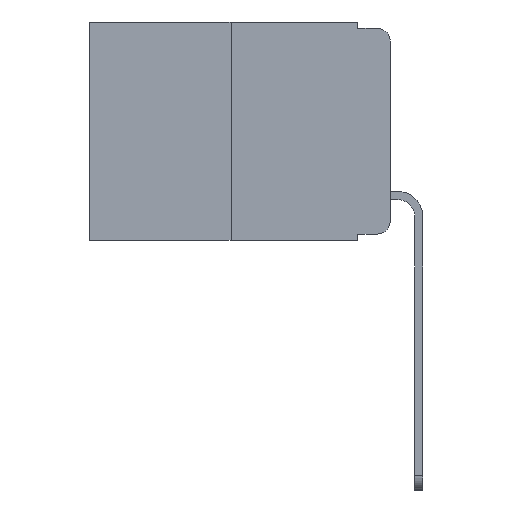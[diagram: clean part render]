
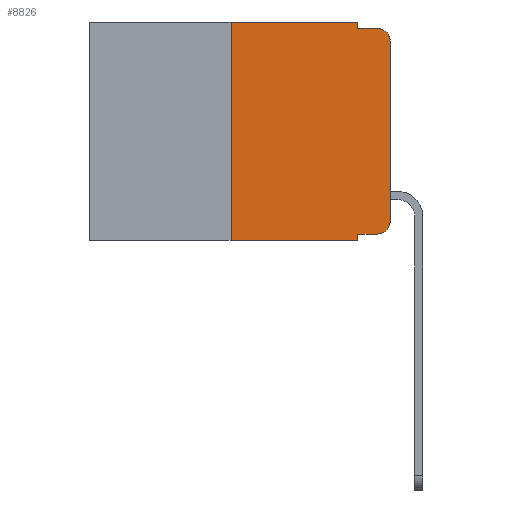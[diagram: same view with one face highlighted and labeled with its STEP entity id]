
A CAD part, left-side view. The second image highlights one B-rep face of the part: STEP entity #8826.
In plain terms, the highlighted planar face has unit normal (-1, 0, 0).
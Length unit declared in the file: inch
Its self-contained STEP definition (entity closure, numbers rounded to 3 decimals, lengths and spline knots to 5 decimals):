
#45 = EDGE_CURVE ( 'NONE', #7923, #2199, #207, .T. ) ;
#149 = CARTESIAN_POINT ( 'NONE',  ( 0., 0.051, -0.01 ) ) ;
#207 = LINE ( 'NONE', #12982, #14011 ) ;
#351 = EDGE_CURVE ( 'NONE', #8322, #7923, #1285, .T. ) ;
#622 = EDGE_CURVE ( 'NONE', #8634, #12331, #730, .T. ) ;
#730 = LINE ( 'NONE', #149, #1102 ) ;
#898 = EDGE_CURVE ( 'NONE', #9922, #12331, #11435, .T. ) ;
#1043 = DIRECTION ( 'NONE',  ( 0., -1., 0. ) ) ;
#1086 = LINE ( 'NONE', #13231, #12305 ) ;
#1102 = VECTOR ( 'NONE', #1043, 39.37008 ) ;
#1285 = LINE ( 'NONE', #11115, #12483 ) ;
#1676 = CARTESIAN_POINT ( 'NONE',  ( 0., 0.02, -0.01 ) ) ;
#1806 = CARTESIAN_POINT ( 'NONE',  ( 0., 0.02, -0.333 ) ) ;
#1904 = LINE ( 'NONE', #10534, #7404 ) ;
#1915 = CARTESIAN_POINT ( 'NONE',  ( 0., 0.051, -0.333 ) ) ;
#2199 = VERTEX_POINT ( 'NONE', #9205 ) ;
#2533 = CARTESIAN_POINT ( 'NONE',  ( 0., 0., 0. ) ) ;
#2540 = CARTESIAN_POINT ( 'NONE',  ( 0., 0.051, -0.01 ) ) ;
#2657 = VERTEX_POINT ( 'NONE', #1806 ) ;
#2938 = EDGE_LOOP ( 'NONE', ( #7087, #11028, #8551, #10740, #12458, #8954, #9771, #4746, #8116, #6561 ) ) ;
#3637 = CARTESIAN_POINT ( 'NONE',  ( 0., 0.051, -0.343 ) ) ;
#3745 = DIRECTION ( 'NONE',  ( 0., 0., 1. ) ) ;
#3995 = CARTESIAN_POINT ( 'NONE',  ( 0., 0.02, -0.313 ) ) ;
#4214 = CARTESIAN_POINT ( 'NONE',  ( 0., 0.051, 0. ) ) ;
#4683 = VECTOR ( 'NONE', #13913, 39.37008 ) ;
#4694 = EDGE_CURVE ( 'NONE', #8322, #13326, #1904, .T. ) ;
#4746 = ORIENTED_EDGE ( 'NONE', *, *, #13057, .F. ) ;
#4862 = CIRCLE ( 'NONE', #6021, 0.02 ) ;
#5087 = PLANE ( 'NONE',  #6906 ) ;
#5114 = DIRECTION ( 'NONE',  ( 0., 0., -1. ) ) ;
#5293 = CARTESIAN_POINT ( 'NONE',  ( 0., 0.25, -0.343 ) ) ;
#5341 = CARTESIAN_POINT ( 'NONE',  ( 0., 0.25, 0. ) ) ;
#5489 = AXIS2_PLACEMENT_3D ( 'NONE', #11499, #9823, #12841 ) ;
#6021 = AXIS2_PLACEMENT_3D ( 'NONE', #3995, #11497, #5114 ) ;
#6042 = VECTOR ( 'NONE', #9025, 39.37008 ) ;
#6199 = DIRECTION ( 'NONE',  ( 0., 0., -1. ) ) ;
#6561 = ORIENTED_EDGE ( 'NONE', *, *, #12378, .T. ) ;
#6906 = AXIS2_PLACEMENT_3D ( 'NONE', #9337, #12574, #6199 ) ;
#7087 = ORIENTED_EDGE ( 'NONE', *, *, #13327, .T. ) ;
#7298 = EDGE_CURVE ( 'NONE', #2199, #8634, #1086, .T. ) ;
#7404 = VECTOR ( 'NONE', #10777, 39.37008 ) ;
#7420 = FACE_OUTER_BOUND ( 'NONE', #2938, .T. ) ;
#7519 = EDGE_CURVE ( 'NONE', #11835, #2657, #9582, .T. ) ;
#7923 = VERTEX_POINT ( 'NONE', #5341 ) ;
#8116 = ORIENTED_EDGE ( 'NONE', *, *, #7519, .T. ) ;
#8322 = VERTEX_POINT ( 'NONE', #5293 ) ;
#8551 = ORIENTED_EDGE ( 'NONE', *, *, #622, .F. ) ;
#8634 = VERTEX_POINT ( 'NONE', #2540 ) ;
#8826 = ADVANCED_FACE ( 'NONE', ( #7420 ), #5087, .F. ) ;
#8855 = VERTEX_POINT ( 'NONE', #13670 ) ;
#8856 = LINE ( 'NONE', #2533, #6042 ) ;
#8954 = ORIENTED_EDGE ( 'NONE', *, *, #351, .F. ) ;
#9025 = DIRECTION ( 'NONE',  ( 0., 0., 1. ) ) ;
#9182 = CARTESIAN_POINT ( 'NONE',  ( 0., 0., -0.03 ) ) ;
#9205 = CARTESIAN_POINT ( 'NONE',  ( 0., 0.051, 0. ) ) ;
#9337 = CARTESIAN_POINT ( 'NONE',  ( 0., 0.473, 0. ) ) ;
#9582 = LINE ( 'NONE', #11220, #12459 ) ;
#9771 = ORIENTED_EDGE ( 'NONE', *, *, #4694, .T. ) ;
#9823 = DIRECTION ( 'NONE',  ( -1., 0., 0. ) ) ;
#9922 = VERTEX_POINT ( 'NONE', #9182 ) ;
#10534 = CARTESIAN_POINT ( 'NONE',  ( 0., 0.473, -0.343 ) ) ;
#10740 = ORIENTED_EDGE ( 'NONE', *, *, #7298, .F. ) ;
#10777 = DIRECTION ( 'NONE',  ( 0., -1., 0. ) ) ;
#11028 = ORIENTED_EDGE ( 'NONE', *, *, #898, .T. ) ;
#11115 = CARTESIAN_POINT ( 'NONE',  ( 0., 0.25, 0. ) ) ;
#11136 = DIRECTION ( 'NONE',  ( 0., 0., -1. ) ) ;
#11220 = CARTESIAN_POINT ( 'NONE',  ( 0., 0.051, -0.333 ) ) ;
#11435 = CIRCLE ( 'NONE', #5489, 0.02 ) ;
#11497 = DIRECTION ( 'NONE',  ( -1., 0., 0. ) ) ;
#11499 = CARTESIAN_POINT ( 'NONE',  ( 0., 0.02, -0.03 ) ) ;
#11835 = VERTEX_POINT ( 'NONE', #1915 ) ;
#12305 = VECTOR ( 'NONE', #11136, 39.37008 ) ;
#12331 = VERTEX_POINT ( 'NONE', #1676 ) ;
#12378 = EDGE_CURVE ( 'NONE', #2657, #8855, #4862, .T. ) ;
#12458 = ORIENTED_EDGE ( 'NONE', *, *, #45, .F. ) ;
#12459 = VECTOR ( 'NONE', #12575, 39.37008 ) ;
#12483 = VECTOR ( 'NONE', #3745, 39.37008 ) ;
#12574 = DIRECTION ( 'NONE',  ( 1., 0., 0. ) ) ;
#12575 = DIRECTION ( 'NONE',  ( 0., -1., 0. ) ) ;
#12607 = DIRECTION ( 'NONE',  ( 0., -1., 0. ) ) ;
#12841 = DIRECTION ( 'NONE',  ( 0., 0., -1. ) ) ;
#12982 = CARTESIAN_POINT ( 'NONE',  ( 0., 0.473, 0. ) ) ;
#13057 = EDGE_CURVE ( 'NONE', #11835, #13326, #13241, .T. ) ;
#13231 = CARTESIAN_POINT ( 'NONE',  ( 0., 0.051, 0. ) ) ;
#13241 = LINE ( 'NONE', #4214, #4683 ) ;
#13326 = VERTEX_POINT ( 'NONE', #3637 ) ;
#13327 = EDGE_CURVE ( 'NONE', #8855, #9922, #8856, .T. ) ;
#13670 = CARTESIAN_POINT ( 'NONE',  ( 0., 0., -0.313 ) ) ;
#13913 = DIRECTION ( 'NONE',  ( 0., 0., -1. ) ) ;
#14011 = VECTOR ( 'NONE', #12607, 39.37008 ) ;
